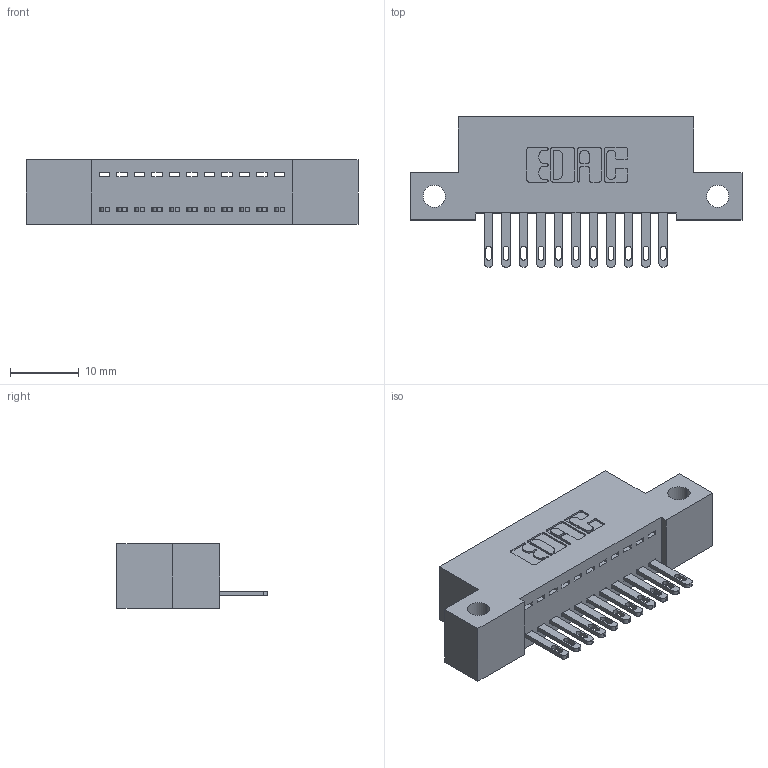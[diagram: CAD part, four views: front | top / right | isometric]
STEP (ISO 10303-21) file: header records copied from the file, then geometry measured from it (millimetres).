
FILE_DESCRIPTION (( 'STEP AP203' ), '1' );
FILE_NAME ('342-011-500-112.STEP', '2018-08-10T14:15:15', ( '' ), ( '' ), 'SwSTEP 2.0', 'SolidWorks 2016', '' );
FILE_SCHEMA (( 'CONFIG_CONTROL_DESIGN' ));
Length unit declared in the file: inch
Products named in the file (3): 342 Part_Side Mount; 345-292-001_345-293-100; 342-011-500-112
Assembly tree (12 placements, depth 2):
  342-011-500-112
    342 Part_Side Mount
    345-292-001_345-293-100  x11
Bounding box: 48.26 x 21.85 x 9.4 mm (x, y, z)
Volume: 4050.1 mm3; surface area: 5227.2 mm2
Topology: 12 solids, 12 shells, 704 faces, 2147 edges, 1430 vertices
Faces by surface type: plane 462, cylinder 242
Entity records: 10535 total; most frequent: CARTESIAN_POINT 1827, ORIENTED_EDGE 1774, DIRECTION 1605, EDGE_CURVE 887, VECTOR 755, LINE 755, VERTEX_POINT 590, AXIS2_PLACEMENT_3D 425
